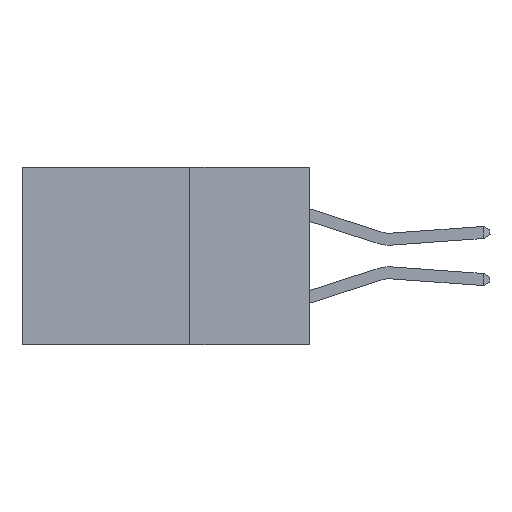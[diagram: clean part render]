
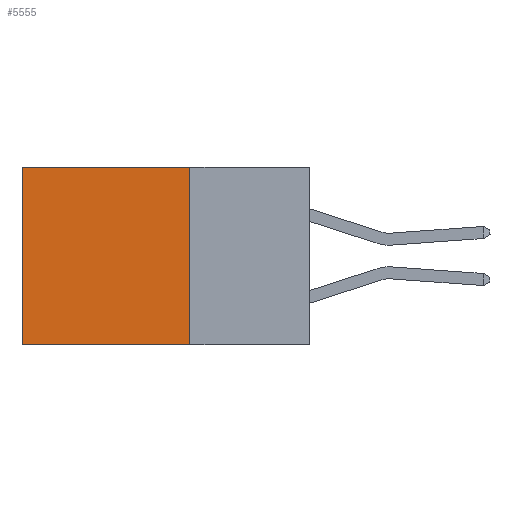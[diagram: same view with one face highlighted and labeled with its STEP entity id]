
A CAD part, left-side view. The second image highlights one B-rep face of the part: STEP entity #5555.
In plain terms, the highlighted planar face has unit normal (-1, 0, 0).
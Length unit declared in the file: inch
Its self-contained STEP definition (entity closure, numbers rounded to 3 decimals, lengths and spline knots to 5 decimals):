
#16 = ORIENTED_EDGE ( 'NONE', *, *, #12499, .F. ) ;
#72 = CARTESIAN_POINT ( 'NONE',  ( 0.298, 0.25, 0. ) ) ;
#278 = CARTESIAN_POINT ( 'NONE',  ( 0.298, 0.25, -0.37 ) ) ;
#1754 = FACE_OUTER_BOUND ( 'NONE', #9180, .T. ) ;
#2238 = VERTEX_POINT ( 'NONE', #4586 ) ;
#2587 = CARTESIAN_POINT ( 'NONE',  ( 0.298, 0.25, -0.37 ) ) ;
#2610 = VECTOR ( 'NONE', #14016, 39.37008 ) ;
#2646 = ORIENTED_EDGE ( 'NONE', *, *, #4615, .F. ) ;
#2749 = DIRECTION ( 'NONE',  ( 0., 1., 0. ) ) ;
#3885 = CARTESIAN_POINT ( 'NONE',  ( 0.298, 0.25, 0. ) ) ;
#4586 = CARTESIAN_POINT ( 'NONE',  ( 0.298, 0.6, 0. ) ) ;
#4615 = EDGE_CURVE ( 'NONE', #11841, #19589, #18195, .T. ) ;
#4826 = AXIS2_PLACEMENT_3D ( 'NONE', #13573, #7802, #18480 ) ;
#5008 = LINE ( 'NONE', #5494, #7805 ) ;
#5494 = CARTESIAN_POINT ( 'NONE',  ( 0.298, 0.6, 0. ) ) ;
#5555 = ADVANCED_FACE ( 'NONE', ( #1754 ), #6285, .F. ) ;
#6285 = PLANE ( 'NONE',  #4826 ) ;
#6551 = VECTOR ( 'NONE', #2749, 39.37008 ) ;
#7802 = DIRECTION ( 'NONE',  ( 1., 0., 0. ) ) ;
#7805 = VECTOR ( 'NONE', #14822, 39.37008 ) ;
#8046 = LINE ( 'NONE', #278, #2610 ) ;
#8861 = CARTESIAN_POINT ( 'NONE',  ( 0.298, 0.25, 0. ) ) ;
#9180 = EDGE_LOOP ( 'NONE', ( #10196, #16, #2646, #14698 ) ) ;
#9507 = VERTEX_POINT ( 'NONE', #12683 ) ;
#10196 = ORIENTED_EDGE ( 'NONE', *, *, #19584, .T. ) ;
#10735 = DIRECTION ( 'NONE',  ( 0., 0., -1. ) ) ;
#11841 = VERTEX_POINT ( 'NONE', #3885 ) ;
#12499 = EDGE_CURVE ( 'NONE', #19589, #9507, #8046, .T. ) ;
#12683 = CARTESIAN_POINT ( 'NONE',  ( 0.298, 0.6, -0.37 ) ) ;
#12688 = LINE ( 'NONE', #8861, #6551 ) ;
#13573 = CARTESIAN_POINT ( 'NONE',  ( 0.298, 0.25, 0. ) ) ;
#14016 = DIRECTION ( 'NONE',  ( 0., 1., 0. ) ) ;
#14698 = ORIENTED_EDGE ( 'NONE', *, *, #15434, .T. ) ;
#14822 = DIRECTION ( 'NONE',  ( 0., 0., -1. ) ) ;
#15434 = EDGE_CURVE ( 'NONE', #11841, #2238, #12688, .T. ) ;
#18195 = LINE ( 'NONE', #72, #18940 ) ;
#18480 = DIRECTION ( 'NONE',  ( 0., 0., -1. ) ) ;
#18940 = VECTOR ( 'NONE', #10735, 39.37008 ) ;
#19584 = EDGE_CURVE ( 'NONE', #2238, #9507, #5008, .T. ) ;
#19589 = VERTEX_POINT ( 'NONE', #2587 ) ;
